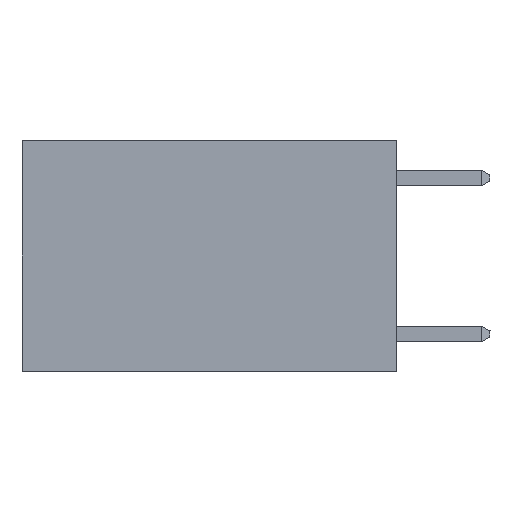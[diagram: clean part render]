
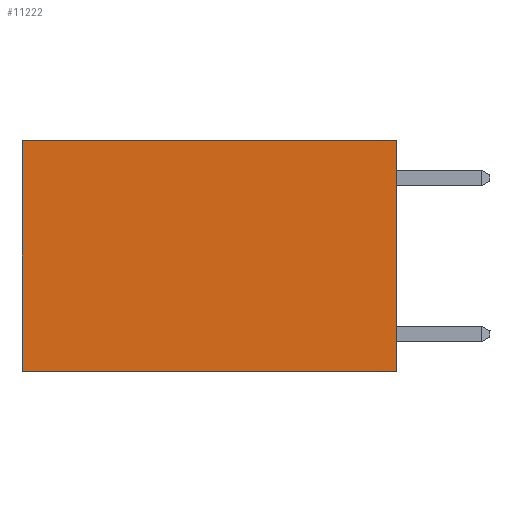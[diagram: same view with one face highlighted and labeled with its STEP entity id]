
A CAD part, left-side view. The second image highlights one B-rep face of the part: STEP entity #11222.
In plain terms, the highlighted planar face has unit normal (-1, 0, 0).
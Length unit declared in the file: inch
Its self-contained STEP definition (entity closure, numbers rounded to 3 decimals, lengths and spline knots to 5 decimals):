
#1415 = FACE_OUTER_BOUND ( 'NONE', #3622, .T. ) ;
#1941 = LINE ( 'NONE', #9549, #8062 ) ;
#3416 = VECTOR ( 'NONE', #10350, 39.37008 ) ;
#3622 = EDGE_LOOP ( 'NONE', ( #14049, #18615, #17789, #17807 ) ) ;
#3975 = CARTESIAN_POINT ( 'NONE',  ( 0.2625, 0.6, 0. ) ) ;
#4007 = VECTOR ( 'NONE', #9983, 39.37008 ) ;
#4119 = LINE ( 'NONE', #18221, #4007 ) ;
#5531 = CARTESIAN_POINT ( 'NONE',  ( 0.2625, 0., 0. ) ) ;
#6010 = DIRECTION ( 'NONE',  ( 1., 0., 0. ) ) ;
#6496 = DIRECTION ( 'NONE',  ( 0., 1., 0. ) ) ;
#8018 = VECTOR ( 'NONE', #6496, 39.37008 ) ;
#8062 = VECTOR ( 'NONE', #11193, 39.37008 ) ;
#8286 = VERTEX_POINT ( 'NONE', #3975 ) ;
#8645 = CARTESIAN_POINT ( 'NONE',  ( 0.2625, 0.6, 0. ) ) ;
#9549 = CARTESIAN_POINT ( 'NONE',  ( 0.2625, 0., -0.37 ) ) ;
#9983 = DIRECTION ( 'NONE',  ( 0., 0., -1. ) ) ;
#10125 = CARTESIAN_POINT ( 'NONE',  ( 0.2625, 0., -0.37 ) ) ;
#10350 = DIRECTION ( 'NONE',  ( 0., 0., -1. ) ) ;
#10599 = AXIS2_PLACEMENT_3D ( 'NONE', #15933, #6010, #17622 ) ;
#10798 = EDGE_CURVE ( 'NONE', #12430, #18797, #4119, .T. ) ;
#11193 = DIRECTION ( 'NONE',  ( 0., 1., 0. ) ) ;
#11222 = ADVANCED_FACE ( 'NONE', ( #1415 ), #12561, .F. ) ;
#12376 = LINE ( 'NONE', #8645, #3416 ) ;
#12430 = VERTEX_POINT ( 'NONE', #5531 ) ;
#12561 = PLANE ( 'NONE',  #10599 ) ;
#12826 = CARTESIAN_POINT ( 'NONE',  ( 0.2625, 0.6, -0.37 ) ) ;
#14049 = ORIENTED_EDGE ( 'NONE', *, *, #15471, .T. ) ;
#14746 = CARTESIAN_POINT ( 'NONE',  ( 0.2625, 0., 0. ) ) ;
#15471 = EDGE_CURVE ( 'NONE', #8286, #16497, #12376, .T. ) ;
#15933 = CARTESIAN_POINT ( 'NONE',  ( 0.2625, 0., 0. ) ) ;
#16497 = VERTEX_POINT ( 'NONE', #12826 ) ;
#17622 = DIRECTION ( 'NONE',  ( 0., 0., -1. ) ) ;
#17789 = ORIENTED_EDGE ( 'NONE', *, *, #10798, .F. ) ;
#17807 = ORIENTED_EDGE ( 'NONE', *, *, #19344, .T. ) ;
#17877 = LINE ( 'NONE', #14746, #8018 ) ;
#18221 = CARTESIAN_POINT ( 'NONE',  ( 0.2625, 0., 0. ) ) ;
#18546 = EDGE_CURVE ( 'NONE', #18797, #16497, #1941, .T. ) ;
#18615 = ORIENTED_EDGE ( 'NONE', *, *, #18546, .F. ) ;
#18797 = VERTEX_POINT ( 'NONE', #10125 ) ;
#19344 = EDGE_CURVE ( 'NONE', #12430, #8286, #17877, .T. ) ;
